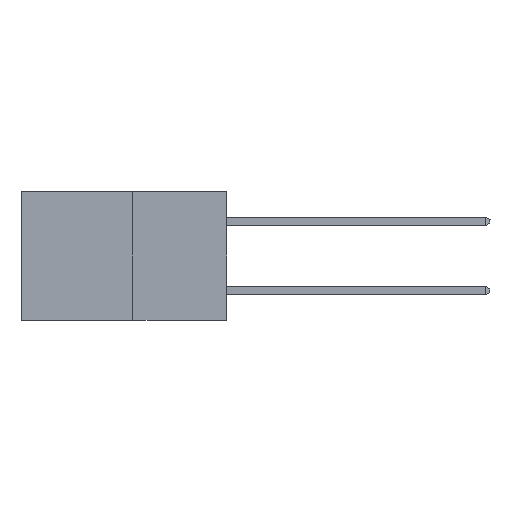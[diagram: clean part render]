
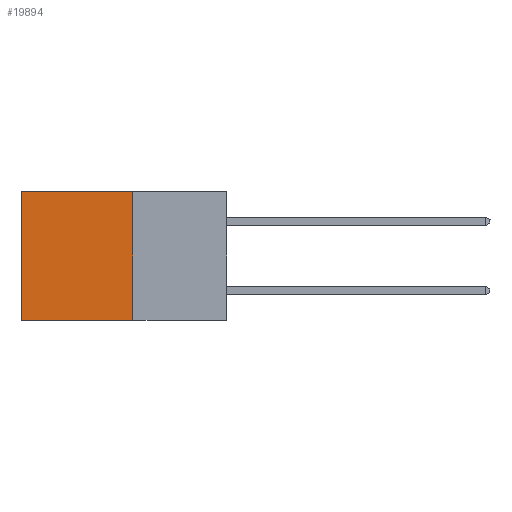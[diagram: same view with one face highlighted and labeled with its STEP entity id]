
A CAD part, left-side view. The second image highlights one B-rep face of the part: STEP entity #19894.
In plain terms, the highlighted planar face has unit normal (-1, 0, 0).
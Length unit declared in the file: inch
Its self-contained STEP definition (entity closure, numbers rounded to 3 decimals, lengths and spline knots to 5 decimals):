
#20 = CARTESIAN_POINT ( 'NONE',  ( 0.277, 0.59, -0.37 ) ) ;
#643 = EDGE_CURVE ( 'NONE', #2684, #17781, #16680, .T. ) ;
#1156 = CARTESIAN_POINT ( 'NONE',  ( 0.277, 0.27, -0.37 ) ) ;
#1260 = EDGE_CURVE ( 'NONE', #7653, #17781, #13651, .T. ) ;
#1414 = VECTOR ( 'NONE', #15716, 39.37008 ) ;
#2470 = LINE ( 'NONE', #1156, #1414 ) ;
#2684 = VERTEX_POINT ( 'NONE', #11918 ) ;
#3747 = DIRECTION ( 'NONE',  ( 0., 1., 0. ) ) ;
#4117 = EDGE_CURVE ( 'NONE', #9530, #7653, #11009, .T. ) ;
#5098 = VECTOR ( 'NONE', #9850, 39.37008 ) ;
#6143 = AXIS2_PLACEMENT_3D ( 'NONE', #18809, #9154, #20410 ) ;
#6515 = ORIENTED_EDGE ( 'NONE', *, *, #1260, .T. ) ;
#6713 = VECTOR ( 'NONE', #10920, 39.37008 ) ;
#7456 = EDGE_LOOP ( 'NONE', ( #6515, #8191, #13481, #19529 ) ) ;
#7653 = VERTEX_POINT ( 'NONE', #8472 ) ;
#8141 = VECTOR ( 'NONE', #3747, 39.37008 ) ;
#8191 = ORIENTED_EDGE ( 'NONE', *, *, #643, .F. ) ;
#8472 = CARTESIAN_POINT ( 'NONE',  ( 0.277, 0.59, 0. ) ) ;
#9154 = DIRECTION ( 'NONE',  ( 1., 0., 0. ) ) ;
#9530 = VERTEX_POINT ( 'NONE', #20455 ) ;
#9850 = DIRECTION ( 'NONE',  ( 0., 0., -1. ) ) ;
#10920 = DIRECTION ( 'NONE',  ( 0., 1., 0. ) ) ;
#11009 = LINE ( 'NONE', #14088, #6713 ) ;
#11918 = CARTESIAN_POINT ( 'NONE',  ( 0.277, 0.27, -0.37 ) ) ;
#12298 = PLANE ( 'NONE',  #6143 ) ;
#13174 = EDGE_CURVE ( 'NONE', #9530, #2684, #2470, .T. ) ;
#13481 = ORIENTED_EDGE ( 'NONE', *, *, #13174, .F. ) ;
#13651 = LINE ( 'NONE', #16721, #5098 ) ;
#14088 = CARTESIAN_POINT ( 'NONE',  ( 0.277, 0.27, 0. ) ) ;
#15716 = DIRECTION ( 'NONE',  ( 0., 0., -1. ) ) ;
#16161 = CARTESIAN_POINT ( 'NONE',  ( 0.277, 0.27, -0.37 ) ) ;
#16680 = LINE ( 'NONE', #16161, #8141 ) ;
#16721 = CARTESIAN_POINT ( 'NONE',  ( 0.277, 0.59, -0.37 ) ) ;
#17781 = VERTEX_POINT ( 'NONE', #20 ) ;
#18809 = CARTESIAN_POINT ( 'NONE',  ( 0.277, 0.27, -0.37 ) ) ;
#19529 = ORIENTED_EDGE ( 'NONE', *, *, #4117, .T. ) ;
#19894 = ADVANCED_FACE ( 'NONE', ( #20214 ), #12298, .F. ) ;
#20214 = FACE_OUTER_BOUND ( 'NONE', #7456, .T. ) ;
#20410 = DIRECTION ( 'NONE',  ( 0., 0., -1. ) ) ;
#20455 = CARTESIAN_POINT ( 'NONE',  ( 0.277, 0.27, 0. ) ) ;
